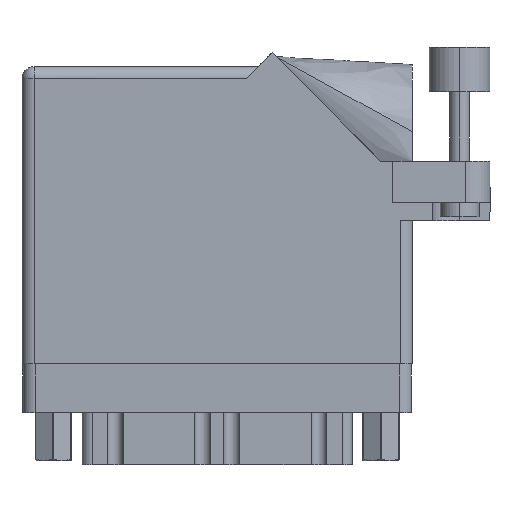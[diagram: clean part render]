
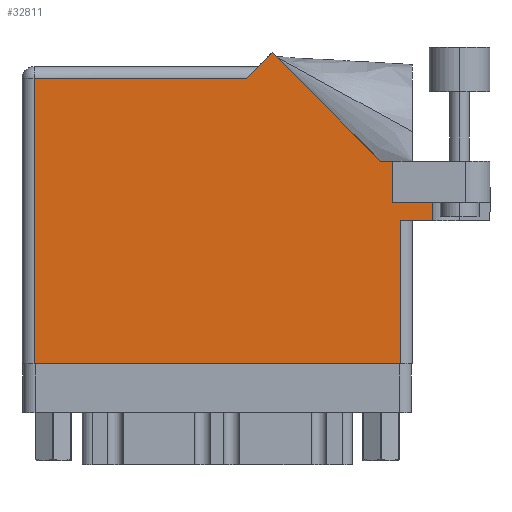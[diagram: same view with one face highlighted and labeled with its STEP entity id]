
A CAD part, front view. The second image highlights one B-rep face of the part: STEP entity #32811.
In plain terms, the highlighted face is planar.
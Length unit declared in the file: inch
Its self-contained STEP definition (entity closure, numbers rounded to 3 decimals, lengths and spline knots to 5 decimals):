
#1898 = CARTESIAN_POINT ( 'NONE',  ( 2.1115, 0.737, 0. ) ) ;
#1904 = LINE ( 'NONE', #13959, #9213 ) ;
#2163 = DIRECTION ( 'NONE',  ( -1., 0., 0. ) ) ;
#2473 = LINE ( 'NONE', #14071, #17880 ) ;
#3705 = CARTESIAN_POINT ( 'NONE',  ( 1.28771, 1.60071, 0. ) ) ;
#3747 = EDGE_CURVE ( 'NONE', #39802, #21865, #43271, .T. ) ;
#4759 = ORIENTED_EDGE ( 'NONE', *, *, #28023, .T. ) ;
#4899 = VERTEX_POINT ( 'NONE', #27122 ) ;
#5212 = VECTOR ( 'NONE', #15146, 39.37008 ) ;
#5258 = LINE ( 'NONE', #22904, #13992 ) ;
#5860 = ORIENTED_EDGE ( 'NONE', *, *, #19805, .F. ) ;
#6754 = ORIENTED_EDGE ( 'NONE', *, *, #16240, .T. ) ;
#7754 = LINE ( 'NONE', #33130, #39534 ) ;
#8465 = ORIENTED_EDGE ( 'NONE', *, *, #3747, .T. ) ;
#8482 = DIRECTION ( 'NONE',  ( 0., 1., 0. ) ) ;
#9197 = CARTESIAN_POINT ( 'NONE',  ( 1.948, 0., 0. ) ) ;
#9213 = VECTOR ( 'NONE', #13501, 39.37008 ) ;
#9601 = VERTEX_POINT ( 'NONE', #24368 ) ;
#9812 = CARTESIAN_POINT ( 'NONE',  ( 0.062, 0., 0. ) ) ;
#9888 = CARTESIAN_POINT ( 'NONE',  ( 2.41, 1.044, 0. ) ) ;
#10172 = VERTEX_POINT ( 'NONE', #9812 ) ;
#10182 = CARTESIAN_POINT ( 'NONE',  ( 1.84442, 1.044, 0. ) ) ;
#10431 = ORIENTED_EDGE ( 'NONE', *, *, #20852, .T. ) ;
#13501 = DIRECTION ( 'NONE',  ( -0.707, -0.707, 0. ) ) ;
#13909 = EDGE_CURVE ( 'NONE', #10172, #43878, #42664, .T. ) ;
#13959 = CARTESIAN_POINT ( 'NONE',  ( 1.217, 1.53, 0. ) ) ;
#13992 = VECTOR ( 'NONE', #34008, 39.37008 ) ;
#14071 = CARTESIAN_POINT ( 'NONE',  ( 1.948, 0.737, 0. ) ) ;
#14498 = CARTESIAN_POINT ( 'NONE',  ( 0., 1.468, 0. ) ) ;
#14761 = ORIENTED_EDGE ( 'NONE', *, *, #26450, .F. ) ;
#15146 = DIRECTION ( 'NONE',  ( 1., 0., 0. ) ) ;
#15654 = ORIENTED_EDGE ( 'NONE', *, *, #46604, .T. ) ;
#16240 = EDGE_CURVE ( 'NONE', #16897, #10172, #24658, .T. ) ;
#16897 = VERTEX_POINT ( 'NONE', #26441 ) ;
#17162 = LINE ( 'NONE', #9888, #37856 ) ;
#17399 = VERTEX_POINT ( 'NONE', #20261 ) ;
#17806 = AXIS2_PLACEMENT_3D ( 'NONE', #33243, #29392, #22623 ) ;
#17880 = VECTOR ( 'NONE', #18577, 39.37008 ) ;
#18498 = EDGE_CURVE ( 'NONE', #43878, #9601, #2473, .T. ) ;
#18545 = LINE ( 'NONE', #45089, #5212 ) ;
#18577 = DIRECTION ( 'NONE',  ( 0., 1., 0. ) ) ;
#18969 = ORIENTED_EDGE ( 'NONE', *, *, #18498, .T. ) ;
#19805 = EDGE_CURVE ( 'NONE', #32048, #46656, #30209, .T. ) ;
#20261 = CARTESIAN_POINT ( 'NONE',  ( 1.91, 0.831, 0. ) ) ;
#20362 = DIRECTION ( 'NONE',  ( 0., -1., 0. ) ) ;
#20852 = EDGE_CURVE ( 'NONE', #17399, #33899, #7754, .T. ) ;
#21865 = VERTEX_POINT ( 'NONE', #3705 ) ;
#22623 = DIRECTION ( 'NONE',  ( -1., 0., 0. ) ) ;
#22904 = CARTESIAN_POINT ( 'NONE',  ( 2.01, 0.737, 0. ) ) ;
#23533 = VECTOR ( 'NONE', #24918, 39.37008 ) ;
#24368 = CARTESIAN_POINT ( 'NONE',  ( 1.948, 0.737, 0. ) ) ;
#24658 = LINE ( 'NONE', #42566, #34952 ) ;
#24918 = DIRECTION ( 'NONE',  ( -0.707, 0.707, 0. ) ) ;
#24945 = EDGE_LOOP ( 'NONE', ( #40705, #18969, #15654, #5860, #14761, #10431, #43713, #8465, #42379, #4759, #6754 ) ) ;
#26304 = VECTOR ( 'NONE', #33118, 39.37008 ) ;
#26441 = CARTESIAN_POINT ( 'NONE',  ( 0.062, 1.468, 0. ) ) ;
#26450 = EDGE_CURVE ( 'NONE', #17399, #32048, #18545, .T. ) ;
#27094 = CARTESIAN_POINT ( 'NONE',  ( 1.91, 1.044, 0. ) ) ;
#27122 = CARTESIAN_POINT ( 'NONE',  ( 1.155, 1.468, 0. ) ) ;
#28023 = EDGE_CURVE ( 'NONE', #4899, #16897, #32845, .T. ) ;
#28808 = VECTOR ( 'NONE', #36567, 39.37008 ) ;
#29224 = DIRECTION ( 'NONE',  ( -1., 0., 0. ) ) ;
#29392 = DIRECTION ( 'NONE',  ( 0., 0., -1. ) ) ;
#30209 = LINE ( 'NONE', #37222, #26304 ) ;
#32048 = VERTEX_POINT ( 'NONE', #37756 ) ;
#32811 = ADVANCED_FACE ( 'NONE', ( #37094 ), #33487, .F. ) ;
#32845 = LINE ( 'NONE', #14498, #41562 ) ;
#33118 = DIRECTION ( 'NONE',  ( 0., -1., 0. ) ) ;
#33130 = CARTESIAN_POINT ( 'NONE',  ( 1.91, 0.831, 0. ) ) ;
#33243 = CARTESIAN_POINT ( 'NONE',  ( 0., 1.53, 0. ) ) ;
#33487 = PLANE ( 'NONE',  #17806 ) ;
#33899 = VERTEX_POINT ( 'NONE', #27094 ) ;
#34008 = DIRECTION ( 'NONE',  ( 1., 0., 0. ) ) ;
#34952 = VECTOR ( 'NONE', #20362, 39.37008 ) ;
#36233 = EDGE_CURVE ( 'NONE', #21865, #4899, #1904, .T. ) ;
#36567 = DIRECTION ( 'NONE',  ( 1., 0., 0. ) ) ;
#37094 = FACE_OUTER_BOUND ( 'NONE', #24945, .T. ) ;
#37222 = CARTESIAN_POINT ( 'NONE',  ( 2.1115, 1.16177, 0. ) ) ;
#37756 = CARTESIAN_POINT ( 'NONE',  ( 2.1115, 0.831, 0. ) ) ;
#37856 = VECTOR ( 'NONE', #2163, 39.37008 ) ;
#39534 = VECTOR ( 'NONE', #8482, 39.37008 ) ;
#39681 = CARTESIAN_POINT ( 'NONE',  ( 1.84442, 1.044, 0. ) ) ;
#39802 = VERTEX_POINT ( 'NONE', #39681 ) ;
#40705 = ORIENTED_EDGE ( 'NONE', *, *, #13909, .T. ) ;
#40913 = CARTESIAN_POINT ( 'NONE',  ( 0., 0., 0. ) ) ;
#41562 = VECTOR ( 'NONE', #29224, 39.37008 ) ;
#42379 = ORIENTED_EDGE ( 'NONE', *, *, #36233, .T. ) ;
#42566 = CARTESIAN_POINT ( 'NONE',  ( 0.062, 0., 0. ) ) ;
#42664 = LINE ( 'NONE', #40913, #28808 ) ;
#43271 = LINE ( 'NONE', #10182, #23533 ) ;
#43713 = ORIENTED_EDGE ( 'NONE', *, *, #45768, .T. ) ;
#43878 = VERTEX_POINT ( 'NONE', #9197 ) ;
#45089 = CARTESIAN_POINT ( 'NONE',  ( 1.91, 0.831, 0. ) ) ;
#45768 = EDGE_CURVE ( 'NONE', #33899, #39802, #17162, .T. ) ;
#46604 = EDGE_CURVE ( 'NONE', #9601, #46656, #5258, .T. ) ;
#46656 = VERTEX_POINT ( 'NONE', #1898 ) ;
